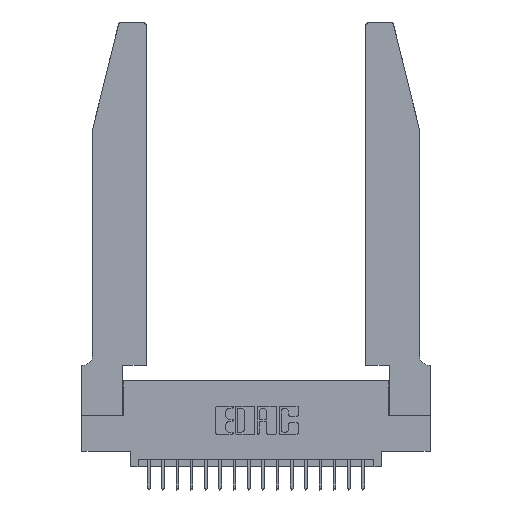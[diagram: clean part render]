
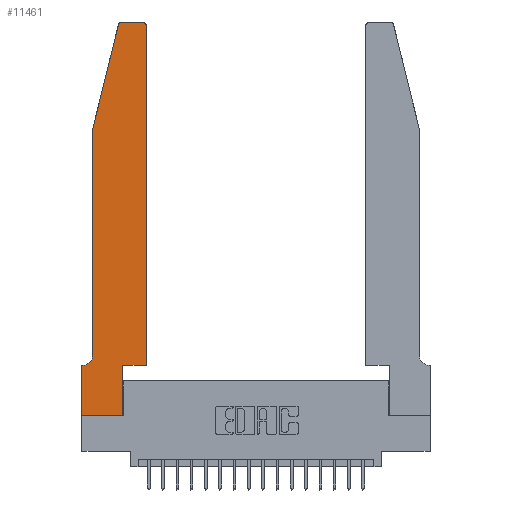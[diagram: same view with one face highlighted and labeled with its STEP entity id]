
A CAD part, top view. The second image highlights one B-rep face of the part: STEP entity #11461.
In plain terms, the highlighted planar face has unit normal (0, 0, 1).
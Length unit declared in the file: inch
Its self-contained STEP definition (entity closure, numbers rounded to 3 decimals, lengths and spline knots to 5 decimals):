
#94 = LINE ( 'NONE', #18228, #3366 ) ;
#213 = CARTESIAN_POINT ( 'NONE',  ( 0.4505, 0.35, 0.37 ) ) ;
#612 = CARTESIAN_POINT ( 'NONE',  ( 0.25487, 2.72718, 0.37 ) ) ;
#684 = ORIENTED_EDGE ( 'NONE', *, *, #16398, .T. ) ;
#871 = DIRECTION ( 'NONE',  ( -0.239, -0.971, 0. ) ) ;
#2390 = LINE ( 'NONE', #19980, #8719 ) ;
#2761 = AXIS2_PLACEMENT_3D ( 'NONE', #11484, #3507, #18144 ) ;
#2839 = CARTESIAN_POINT ( 'NONE',  ( 0.4505, 2.72, 0.37 ) ) ;
#3121 = FACE_OUTER_BOUND ( 'NONE', #16209, .T. ) ;
#3197 = ORIENTED_EDGE ( 'NONE', *, *, #7357, .T. ) ;
#3366 = VECTOR ( 'NONE', #11702, 39.37008 ) ;
#3371 = CARTESIAN_POINT ( 'NONE',  ( 0.2865, 0.35, 0.37 ) ) ;
#3507 = DIRECTION ( 'NONE',  ( 0., 0., 1. ) ) ;
#4023 = VERTEX_POINT ( 'NONE', #2839 ) ;
#4243 = LINE ( 'NONE', #17585, #15924 ) ;
#4585 = EDGE_CURVE ( 'NONE', #6282, #6614, #4243, .T. ) ;
#4960 = EDGE_CURVE ( 'NONE', #6614, #14224, #14383, .T. ) ;
#5062 = ORIENTED_EDGE ( 'NONE', *, *, #9828, .T. ) ;
#5221 = CARTESIAN_POINT ( 'NONE',  ( 0.284, 2.72, 0.37 ) ) ;
#5285 = DIRECTION ( 'NONE',  ( 0., 0., 1. ) ) ;
#5338 = DIRECTION ( 'NONE',  ( 0., 1., 0. ) ) ;
#5398 = CARTESIAN_POINT ( 'NONE',  ( 0.0055, 0.42, 0.37 ) ) ;
#5466 = VECTOR ( 'NONE', #9842, 39.37008 ) ;
#5690 = LINE ( 'NONE', #13935, #8972 ) ;
#5784 = DIRECTION ( 'NONE',  ( -1., 0., 0. ) ) ;
#5942 = CARTESIAN_POINT ( 'NONE',  ( 0.4505, 0.35, 0.37 ) ) ;
#5983 = ORIENTED_EDGE ( 'NONE', *, *, #11140, .T. ) ;
#6177 = CARTESIAN_POINT ( 'NONE',  ( 0.2865, 0., 0.37 ) ) ;
#6211 = CIRCLE ( 'NONE', #16597, 0.03 ) ;
#6282 = VERTEX_POINT ( 'NONE', #15436 ) ;
#6292 = ORIENTED_EDGE ( 'NONE', *, *, #4585, .T. ) ;
#6335 = CARTESIAN_POINT ( 'NONE',  ( 0., 0., 0.37 ) ) ;
#6430 = CARTESIAN_POINT ( 'NONE',  ( 0.4205, 2.75, 0.37 ) ) ;
#6547 = DIRECTION ( 'NONE',  ( 1., 0., 0. ) ) ;
#6614 = VERTEX_POINT ( 'NONE', #12597 ) ;
#6985 = EDGE_CURVE ( 'NONE', #12883, #14653, #2390, .T. ) ;
#7357 = EDGE_CURVE ( 'NONE', #11469, #19571, #12209, .T. ) ;
#7405 = ORIENTED_EDGE ( 'NONE', *, *, #13566, .T. ) ;
#7759 = DIRECTION ( 'NONE',  ( 0., 0., 1. ) ) ;
#8584 = VECTOR ( 'NONE', #13292, 39.37008 ) ;
#8719 = VECTOR ( 'NONE', #871, 39.37008 ) ;
#8972 = VECTOR ( 'NONE', #5784, 39.37008 ) ;
#9051 = EDGE_CURVE ( 'NONE', #14653, #11469, #12024, .T. ) ;
#9118 = VECTOR ( 'NONE', #11084, 39.37008 ) ;
#9544 = CARTESIAN_POINT ( 'NONE',  ( 0.2865, 0.35, 0.37 ) ) ;
#9775 = AXIS2_PLACEMENT_3D ( 'NONE', #10877, #7759, #14448 ) ;
#9828 = EDGE_CURVE ( 'NONE', #19177, #17590, #5690, .T. ) ;
#9842 = DIRECTION ( 'NONE',  ( 0., -1., 0. ) ) ;
#10050 = VERTEX_POINT ( 'NONE', #3371 ) ;
#10534 = EDGE_CURVE ( 'NONE', #4023, #19177, #12006, .T. ) ;
#10718 = ORIENTED_EDGE ( 'NONE', *, *, #6985, .T. ) ;
#10877 = CARTESIAN_POINT ( 'NONE',  ( 0.4205, 2.72, 0.37 ) ) ;
#10969 = VECTOR ( 'NONE', #5338, 39.37008 ) ;
#11084 = DIRECTION ( 'NONE',  ( 0., 1., 0. ) ) ;
#11140 = EDGE_CURVE ( 'NONE', #19571, #6282, #94, .T. ) ;
#11337 = ORIENTED_EDGE ( 'NONE', *, *, #19081, .T. ) ;
#11461 = ADVANCED_FACE ( 'NONE', ( #3121 ), #15070, .T. ) ;
#11469 = VERTEX_POINT ( 'NONE', #13350 ) ;
#11484 = CARTESIAN_POINT ( 'NONE',  ( 0., 0.35, 0.37 ) ) ;
#11702 = DIRECTION ( 'NONE',  ( -1., 0., 0. ) ) ;
#12006 = CIRCLE ( 'NONE', #9775, 0.03 ) ;
#12024 = LINE ( 'NONE', #14625, #5466 ) ;
#12029 = DIRECTION ( 'NONE',  ( 0., 0., -1. ) ) ;
#12174 = DIRECTION ( 'NONE',  ( -1., 0., 0. ) ) ;
#12209 = CIRCLE ( 'NONE', #18613, 0.07 ) ;
#12597 = CARTESIAN_POINT ( 'NONE',  ( 0., 0., 0.37 ) ) ;
#12883 = VERTEX_POINT ( 'NONE', #612 ) ;
#13276 = DIRECTION ( 'NONE',  ( 1., 0., 0. ) ) ;
#13292 = DIRECTION ( 'NONE',  ( 1., 0., 0. ) ) ;
#13350 = CARTESIAN_POINT ( 'NONE',  ( 0.0755, 0.42, 0.37 ) ) ;
#13566 = EDGE_CURVE ( 'NONE', #10050, #16160, #19779, .T. ) ;
#13677 = ORIENTED_EDGE ( 'NONE', *, *, #9051, .T. ) ;
#13910 = ORIENTED_EDGE ( 'NONE', *, *, #17218, .T. ) ;
#13935 = CARTESIAN_POINT ( 'NONE',  ( 0.2605, 2.75, 0.37 ) ) ;
#14224 = VERTEX_POINT ( 'NONE', #6177 ) ;
#14383 = LINE ( 'NONE', #6335, #15128 ) ;
#14448 = DIRECTION ( 'NONE',  ( 1., 0., 0. ) ) ;
#14625 = CARTESIAN_POINT ( 'NONE',  ( 0.0755, 2., 0.37 ) ) ;
#14653 = VERTEX_POINT ( 'NONE', #19807 ) ;
#14773 = ORIENTED_EDGE ( 'NONE', *, *, #4960, .T. ) ;
#15070 = PLANE ( 'NONE',  #2761 ) ;
#15128 = VECTOR ( 'NONE', #6547, 39.37008 ) ;
#15367 = CARTESIAN_POINT ( 'NONE',  ( 0.0055, 0.35, 0.37 ) ) ;
#15436 = CARTESIAN_POINT ( 'NONE',  ( 0., 0.35, 0.37 ) ) ;
#15924 = VECTOR ( 'NONE', #16848, 39.37008 ) ;
#16160 = VERTEX_POINT ( 'NONE', #5942 ) ;
#16209 = EDGE_LOOP ( 'NONE', ( #5062, #684, #10718, #13677, #3197, #5983, #6292, #14773, #11337, #7405, #13910, #16613 ) ) ;
#16398 = EDGE_CURVE ( 'NONE', #17590, #12883, #6211, .T. ) ;
#16597 = AXIS2_PLACEMENT_3D ( 'NONE', #5221, #5285, #13276 ) ;
#16613 = ORIENTED_EDGE ( 'NONE', *, *, #10534, .T. ) ;
#16848 = DIRECTION ( 'NONE',  ( 0., -1., 0. ) ) ;
#17218 = EDGE_CURVE ( 'NONE', #16160, #4023, #19409, .T. ) ;
#17585 = CARTESIAN_POINT ( 'NONE',  ( 0., 0., 0.37 ) ) ;
#17590 = VERTEX_POINT ( 'NONE', #17674 ) ;
#17674 = CARTESIAN_POINT ( 'NONE',  ( 0.284, 2.75, 0.37 ) ) ;
#18144 = DIRECTION ( 'NONE',  ( 1., 0., 0. ) ) ;
#18228 = CARTESIAN_POINT ( 'NONE',  ( 0.0755, 0.35, 0.37 ) ) ;
#18613 = AXIS2_PLACEMENT_3D ( 'NONE', #5398, #12029, #12174 ) ;
#19081 = EDGE_CURVE ( 'NONE', #14224, #10050, #20844, .T. ) ;
#19177 = VERTEX_POINT ( 'NONE', #6430 ) ;
#19409 = LINE ( 'NONE', #20118, #10969 ) ;
#19571 = VERTEX_POINT ( 'NONE', #15367 ) ;
#19779 = LINE ( 'NONE', #213, #8584 ) ;
#19807 = CARTESIAN_POINT ( 'NONE',  ( 0.0755, 2., 0.37 ) ) ;
#19980 = CARTESIAN_POINT ( 'NONE',  ( 0.0755, 2., 0.37 ) ) ;
#20118 = CARTESIAN_POINT ( 'NONE',  ( 0.4505, 0.35, 0.37 ) ) ;
#20844 = LINE ( 'NONE', #9544, #9118 ) ;
